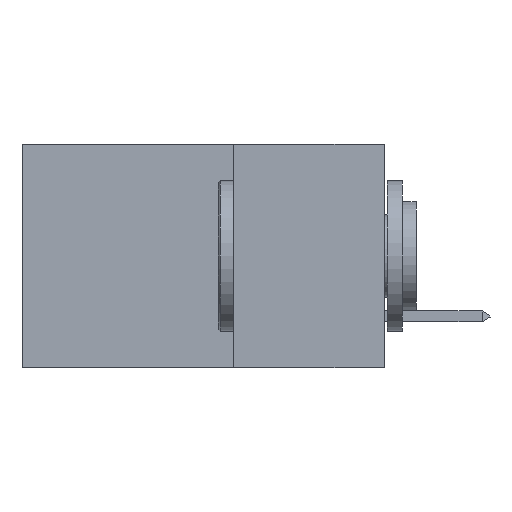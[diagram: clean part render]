
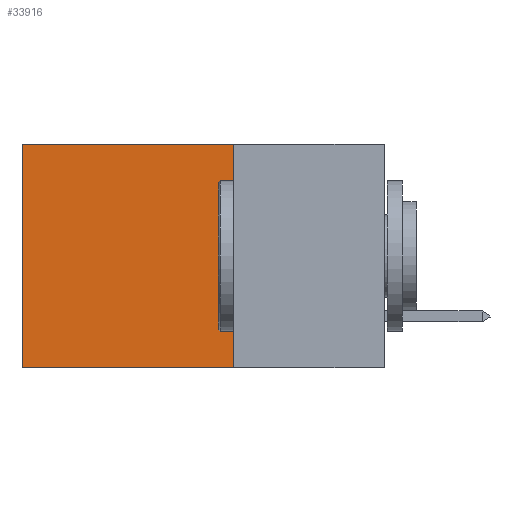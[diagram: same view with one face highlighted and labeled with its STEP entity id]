
A CAD part, left-side view. The second image highlights one B-rep face of the part: STEP entity #33916.
In plain terms, the highlighted planar face has unit normal (-1, 0, 0).
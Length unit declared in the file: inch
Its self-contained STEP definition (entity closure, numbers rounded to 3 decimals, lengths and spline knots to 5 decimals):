
#1212 = DIRECTION ( 'NONE',  ( 0., 1., 0. ) ) ;
#3462 = EDGE_CURVE ( 'NONE', #26191, #26093, #7813, .T. ) ;
#3634 = ORIENTED_EDGE ( 'NONE', *, *, #19938, .T. ) ;
#7408 = VECTOR ( 'NONE', #34708, 39.37008 ) ;
#7813 = LINE ( 'NONE', #30657, #36273 ) ;
#7943 = EDGE_LOOP ( 'NONE', ( #3634, #41535, #12476, #35274 ) ) ;
#8903 = CARTESIAN_POINT ( 'NONE',  ( 0.2875, 0.25, -0.37 ) ) ;
#9439 = CARTESIAN_POINT ( 'NONE',  ( 0.2875, 0.25, 0. ) ) ;
#10111 = CARTESIAN_POINT ( 'NONE',  ( 0.2875, 0.6, -0.37 ) ) ;
#11995 = EDGE_CURVE ( 'NONE', #26191, #41980, #49061, .T. ) ;
#12476 = ORIENTED_EDGE ( 'NONE', *, *, #3462, .F. ) ;
#17055 = CARTESIAN_POINT ( 'NONE',  ( 0.2875, 0.25, 0. ) ) ;
#17585 = DIRECTION ( 'NONE',  ( 0., 1., 0. ) ) ;
#19226 = DIRECTION ( 'NONE',  ( 0., 0., -1. ) ) ;
#19354 = LINE ( 'NONE', #23990, #33077 ) ;
#19938 = EDGE_CURVE ( 'NONE', #41980, #47887, #25187, .T. ) ;
#23646 = EDGE_CURVE ( 'NONE', #26093, #47887, #19354, .T. ) ;
#23990 = CARTESIAN_POINT ( 'NONE',  ( 0.2875, 0.25, -0.37 ) ) ;
#24168 = FACE_OUTER_BOUND ( 'NONE', #7943, .T. ) ;
#25187 = LINE ( 'NONE', #41474, #7408 ) ;
#26093 = VERTEX_POINT ( 'NONE', #8903 ) ;
#26191 = VERTEX_POINT ( 'NONE', #35114 ) ;
#28530 = DIRECTION ( 'NONE',  ( 1., 0., 0. ) ) ;
#30657 = CARTESIAN_POINT ( 'NONE',  ( 0.2875, 0.25, 0. ) ) ;
#31669 = DIRECTION ( 'NONE',  ( 0., 0., -1. ) ) ;
#31692 = CARTESIAN_POINT ( 'NONE',  ( 0.2875, 0.6, 0. ) ) ;
#31845 = PLANE ( 'NONE',  #39498 ) ;
#33077 = VECTOR ( 'NONE', #1212, 39.37008 ) ;
#33916 = ADVANCED_FACE ( 'NONE', ( #24168 ), #31845, .F. ) ;
#34708 = DIRECTION ( 'NONE',  ( 0., 0., -1. ) ) ;
#35114 = CARTESIAN_POINT ( 'NONE',  ( 0.2875, 0.25, 0. ) ) ;
#35274 = ORIENTED_EDGE ( 'NONE', *, *, #11995, .T. ) ;
#35939 = VECTOR ( 'NONE', #17585, 39.37008 ) ;
#36273 = VECTOR ( 'NONE', #19226, 39.37008 ) ;
#39498 = AXIS2_PLACEMENT_3D ( 'NONE', #9439, #28530, #31669 ) ;
#41474 = CARTESIAN_POINT ( 'NONE',  ( 0.2875, 0.6, 0. ) ) ;
#41535 = ORIENTED_EDGE ( 'NONE', *, *, #23646, .F. ) ;
#41980 = VERTEX_POINT ( 'NONE', #31692 ) ;
#47887 = VERTEX_POINT ( 'NONE', #10111 ) ;
#49061 = LINE ( 'NONE', #17055, #35939 ) ;
